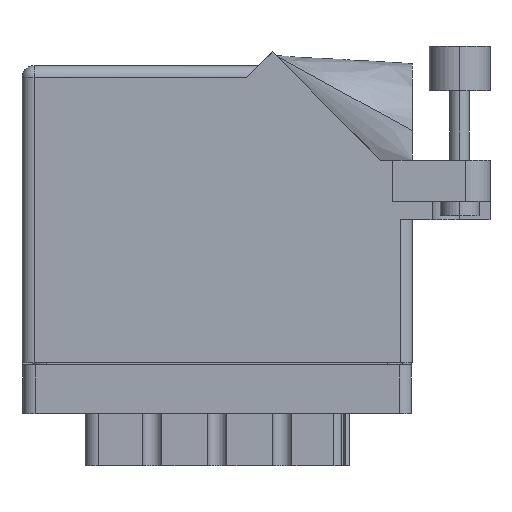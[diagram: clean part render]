
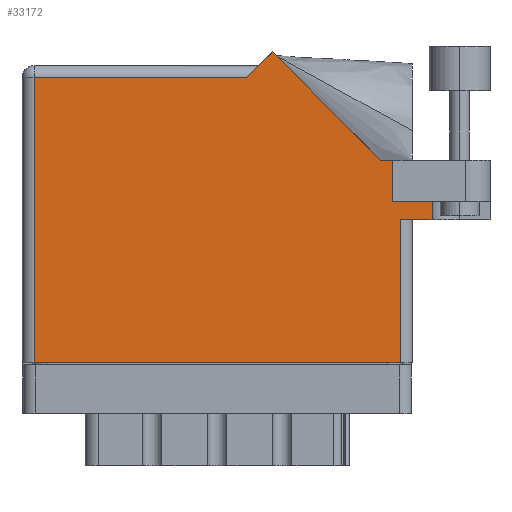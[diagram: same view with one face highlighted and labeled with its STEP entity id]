
A CAD part, front view. The second image highlights one B-rep face of the part: STEP entity #33172.
In plain terms, the highlighted face is planar.
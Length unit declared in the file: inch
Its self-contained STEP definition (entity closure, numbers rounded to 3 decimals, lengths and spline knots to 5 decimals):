
#182 = DIRECTION ( 'NONE',  ( -1., 0., 0. ) ) ;
#511 = DIRECTION ( 'NONE',  ( 0., 1., 0. ) ) ;
#565 = CARTESIAN_POINT ( 'NONE',  ( 0., 0., 0. ) ) ;
#726 = LINE ( 'NONE', #26425, #34368 ) ;
#1202 = CARTESIAN_POINT ( 'NONE',  ( 1.91, 0.831, 0. ) ) ;
#3418 = CARTESIAN_POINT ( 'NONE',  ( 1.948, 0.737, 0. ) ) ;
#3583 = CARTESIAN_POINT ( 'NONE',  ( 0.062, 1.468, 0. ) ) ;
#3654 = VECTOR ( 'NONE', #511, 39.37008 ) ;
#3863 = CARTESIAN_POINT ( 'NONE',  ( 2.1115, 0.737, 0. ) ) ;
#3924 = VERTEX_POINT ( 'NONE', #20169 ) ;
#4011 = EDGE_CURVE ( 'NONE', #14267, #16592, #17440, .T. ) ;
#4409 = ORIENTED_EDGE ( 'NONE', *, *, #27058, .T. ) ;
#5177 = CARTESIAN_POINT ( 'NONE',  ( 1.217, 1.53, 0. ) ) ;
#5481 = LINE ( 'NONE', #25756, #15045 ) ;
#5657 = VECTOR ( 'NONE', #35596, 39.37008 ) ;
#5803 = ORIENTED_EDGE ( 'NONE', *, *, #36638, .T. ) ;
#6556 = VERTEX_POINT ( 'NONE', #22997 ) ;
#6756 = EDGE_CURVE ( 'NONE', #16592, #19328, #18147, .T. ) ;
#7058 = DIRECTION ( 'NONE',  ( 1., 0., 0. ) ) ;
#7483 = CARTESIAN_POINT ( 'NONE',  ( 0., 1.468, 0. ) ) ;
#7767 = VERTEX_POINT ( 'NONE', #3863 ) ;
#7927 = LINE ( 'NONE', #5177, #30205 ) ;
#8225 = DIRECTION ( 'NONE',  ( -0.707, 0.707, 0. ) ) ;
#8459 = EDGE_LOOP ( 'NONE', ( #32239, #10172, #15956, #9103, #8478, #18210, #5803, #17277, #4409, #26317, #13706 ) ) ;
#8478 = ORIENTED_EDGE ( 'NONE', *, *, #35470, .F. ) ;
#9103 = ORIENTED_EDGE ( 'NONE', *, *, #15792, .F. ) ;
#9310 = EDGE_CURVE ( 'NONE', #6556, #3924, #10225, .T. ) ;
#9553 = DIRECTION ( 'NONE',  ( 1., 0., 0. ) ) ;
#9821 = LINE ( 'NONE', #16098, #20668 ) ;
#10172 = ORIENTED_EDGE ( 'NONE', *, *, #12274, .T. ) ;
#10225 = LINE ( 'NONE', #1202, #5657 ) ;
#10673 = LINE ( 'NONE', #34951, #13409 ) ;
#11858 = CARTESIAN_POINT ( 'NONE',  ( 1.155, 1.468, 0. ) ) ;
#12273 = VERTEX_POINT ( 'NONE', #26102 ) ;
#12274 = EDGE_CURVE ( 'NONE', #19328, #28347, #30005, .T. ) ;
#13409 = VECTOR ( 'NONE', #26326, 39.37008 ) ;
#13706 = ORIENTED_EDGE ( 'NONE', *, *, #4011, .T. ) ;
#14267 = VERTEX_POINT ( 'NONE', #3583 ) ;
#14899 = DIRECTION ( 'NONE',  ( 0., -1., 0. ) ) ;
#14926 = LINE ( 'NONE', #26751, #37637 ) ;
#15045 = VECTOR ( 'NONE', #8225, 39.37008 ) ;
#15246 = DIRECTION ( 'NONE',  ( -1., 0., 0. ) ) ;
#15403 = CARTESIAN_POINT ( 'NONE',  ( 0.062, 0., 0. ) ) ;
#15696 = DIRECTION ( 'NONE',  ( 1., 0., 0. ) ) ;
#15792 = EDGE_CURVE ( 'NONE', #12273, #7767, #10673, .T. ) ;
#15932 = VECTOR ( 'NONE', #9553, 39.37008 ) ;
#15956 = ORIENTED_EDGE ( 'NONE', *, *, #25722, .T. ) ;
#16098 = CARTESIAN_POINT ( 'NONE',  ( 2.01, 0.737, 0. ) ) ;
#16235 = AXIS2_PLACEMENT_3D ( 'NONE', #23236, #31788, #182 ) ;
#16592 = VERTEX_POINT ( 'NONE', #18104 ) ;
#16853 = DIRECTION ( 'NONE',  ( -0.707, -0.707, 0. ) ) ;
#17262 = CARTESIAN_POINT ( 'NONE',  ( 1.948, 0.737, 0. ) ) ;
#17277 = ORIENTED_EDGE ( 'NONE', *, *, #28964, .T. ) ;
#17440 = LINE ( 'NONE', #15403, #20585 ) ;
#18104 = CARTESIAN_POINT ( 'NONE',  ( 0.062, 0., 0. ) ) ;
#18147 = LINE ( 'NONE', #565, #15932 ) ;
#18210 = ORIENTED_EDGE ( 'NONE', *, *, #9310, .T. ) ;
#18813 = CARTESIAN_POINT ( 'NONE',  ( 1.28771, 1.60071, 0. ) ) ;
#19328 = VERTEX_POINT ( 'NONE', #37330 ) ;
#19631 = DIRECTION ( 'NONE',  ( -1., 0., 0. ) ) ;
#19945 = VERTEX_POINT ( 'NONE', #34594 ) ;
#20023 = VERTEX_POINT ( 'NONE', #11858 ) ;
#20169 = CARTESIAN_POINT ( 'NONE',  ( 1.91, 1.044, 0. ) ) ;
#20585 = VECTOR ( 'NONE', #14899, 39.37008 ) ;
#20611 = VECTOR ( 'NONE', #19631, 39.37008 ) ;
#20668 = VECTOR ( 'NONE', #7058, 39.37008 ) ;
#21425 = FACE_OUTER_BOUND ( 'NONE', #8459, .T. ) ;
#22997 = CARTESIAN_POINT ( 'NONE',  ( 1.91, 0.831, 0. ) ) ;
#23236 = CARTESIAN_POINT ( 'NONE',  ( 0., 1.53, 0. ) ) ;
#25722 = EDGE_CURVE ( 'NONE', #28347, #7767, #9821, .T. ) ;
#25756 = CARTESIAN_POINT ( 'NONE',  ( 1.84442, 1.044, 0. ) ) ;
#26102 = CARTESIAN_POINT ( 'NONE',  ( 2.1115, 0.831, 0. ) ) ;
#26317 = ORIENTED_EDGE ( 'NONE', *, *, #31237, .T. ) ;
#26326 = DIRECTION ( 'NONE',  ( 0., -1., 0. ) ) ;
#26425 = CARTESIAN_POINT ( 'NONE',  ( 2.41, 1.044, 0. ) ) ;
#26751 = CARTESIAN_POINT ( 'NONE',  ( 1.91, 0.831, 0. ) ) ;
#27058 = EDGE_CURVE ( 'NONE', #27479, #20023, #7927, .T. ) ;
#27479 = VERTEX_POINT ( 'NONE', #18813 ) ;
#28347 = VERTEX_POINT ( 'NONE', #17262 ) ;
#28964 = EDGE_CURVE ( 'NONE', #19945, #27479, #5481, .T. ) ;
#30005 = LINE ( 'NONE', #3418, #3654 ) ;
#30205 = VECTOR ( 'NONE', #16853, 39.37008 ) ;
#30221 = LINE ( 'NONE', #7483, #20611 ) ;
#31237 = EDGE_CURVE ( 'NONE', #20023, #14267, #30221, .T. ) ;
#31788 = DIRECTION ( 'NONE',  ( 0., 0., -1. ) ) ;
#32239 = ORIENTED_EDGE ( 'NONE', *, *, #6756, .T. ) ;
#33172 = ADVANCED_FACE ( 'NONE', ( #21425 ), #34576, .F. ) ;
#34368 = VECTOR ( 'NONE', #15246, 39.37008 ) ;
#34576 = PLANE ( 'NONE',  #16235 ) ;
#34594 = CARTESIAN_POINT ( 'NONE',  ( 1.84442, 1.044, 0. ) ) ;
#34951 = CARTESIAN_POINT ( 'NONE',  ( 2.1115, 1.16177, 0. ) ) ;
#35470 = EDGE_CURVE ( 'NONE', #6556, #12273, #14926, .T. ) ;
#35596 = DIRECTION ( 'NONE',  ( 0., 1., 0. ) ) ;
#36638 = EDGE_CURVE ( 'NONE', #3924, #19945, #726, .T. ) ;
#37330 = CARTESIAN_POINT ( 'NONE',  ( 1.948, 0., 0. ) ) ;
#37637 = VECTOR ( 'NONE', #15696, 39.37008 ) ;
